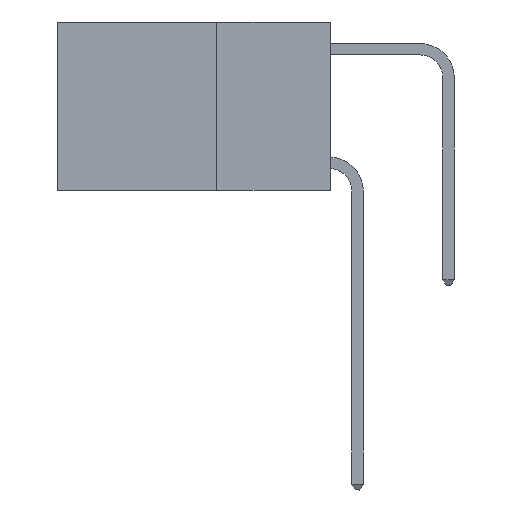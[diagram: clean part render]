
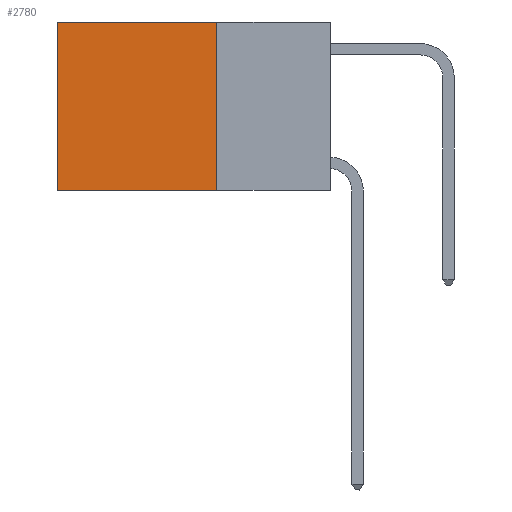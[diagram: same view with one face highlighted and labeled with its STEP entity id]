
A CAD part, left-side view. The second image highlights one B-rep face of the part: STEP entity #2780.
In plain terms, the highlighted planar face has unit normal (-1, 0, 0).
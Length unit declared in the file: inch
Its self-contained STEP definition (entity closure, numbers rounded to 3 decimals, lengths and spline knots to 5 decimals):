
#65 = ORIENTED_EDGE ( 'NONE', *, *, #18686, .T. ) ;
#1254 = CARTESIAN_POINT ( 'NONE',  ( 0.2625, 0.25, -0.37 ) ) ;
#2780 = ADVANCED_FACE ( 'NONE', ( #5584 ), #19964, .F. ) ;
#3074 = EDGE_CURVE ( 'NONE', #12202, #26096, #26659, .T. ) ;
#3078 = DIRECTION ( 'NONE',  ( 0., 0., -1. ) ) ;
#3370 = EDGE_CURVE ( 'NONE', #12202, #13788, #7608, .T. ) ;
#3902 = ORIENTED_EDGE ( 'NONE', *, *, #3074, .T. ) ;
#5314 = DIRECTION ( 'NONE',  ( 0., 0., -1. ) ) ;
#5584 = FACE_OUTER_BOUND ( 'NONE', #10580, .T. ) ;
#5768 = VERTEX_POINT ( 'NONE', #17823 ) ;
#5908 = CARTESIAN_POINT ( 'NONE',  ( 0.2625, 0.25, 0. ) ) ;
#6244 = CARTESIAN_POINT ( 'NONE',  ( 0.2625, 0.25, 0. ) ) ;
#6711 = VECTOR ( 'NONE', #3078, 39.37008 ) ;
#7608 = LINE ( 'NONE', #26071, #6711 ) ;
#8458 = DIRECTION ( 'NONE',  ( 0., 1., 0. ) ) ;
#8736 = DIRECTION ( 'NONE',  ( 0., 1., 0. ) ) ;
#9994 = ORIENTED_EDGE ( 'NONE', *, *, #18735, .F. ) ;
#10580 = EDGE_LOOP ( 'NONE', ( #65, #9994, #17799, #3902 ) ) ;
#10778 = LINE ( 'NONE', #16704, #16015 ) ;
#12202 = VERTEX_POINT ( 'NONE', #5908 ) ;
#12703 = CARTESIAN_POINT ( 'NONE',  ( 0.2625, 0.6, 0. ) ) ;
#12802 = VECTOR ( 'NONE', #8458, 39.37008 ) ;
#13359 = VECTOR ( 'NONE', #20767, 39.37008 ) ;
#13788 = VERTEX_POINT ( 'NONE', #1254 ) ;
#16015 = VECTOR ( 'NONE', #8736, 39.37008 ) ;
#16704 = CARTESIAN_POINT ( 'NONE',  ( 0.2625, 0.25, -0.37 ) ) ;
#17743 = CARTESIAN_POINT ( 'NONE',  ( 0.2625, 0.6, 0. ) ) ;
#17799 = ORIENTED_EDGE ( 'NONE', *, *, #3370, .F. ) ;
#17823 = CARTESIAN_POINT ( 'NONE',  ( 0.2625, 0.6, -0.37 ) ) ;
#17942 = CARTESIAN_POINT ( 'NONE',  ( 0.2625, 0.25, 0. ) ) ;
#18686 = EDGE_CURVE ( 'NONE', #26096, #5768, #23083, .T. ) ;
#18735 = EDGE_CURVE ( 'NONE', #13788, #5768, #10778, .T. ) ;
#19964 = PLANE ( 'NONE',  #20187 ) ;
#20187 = AXIS2_PLACEMENT_3D ( 'NONE', #17942, #26381, #5314 ) ;
#20767 = DIRECTION ( 'NONE',  ( 0., 0., -1. ) ) ;
#23083 = LINE ( 'NONE', #12703, #13359 ) ;
#26071 = CARTESIAN_POINT ( 'NONE',  ( 0.2625, 0.25, 0. ) ) ;
#26096 = VERTEX_POINT ( 'NONE', #17743 ) ;
#26381 = DIRECTION ( 'NONE',  ( 1., 0., 0. ) ) ;
#26659 = LINE ( 'NONE', #6244, #12802 ) ;
